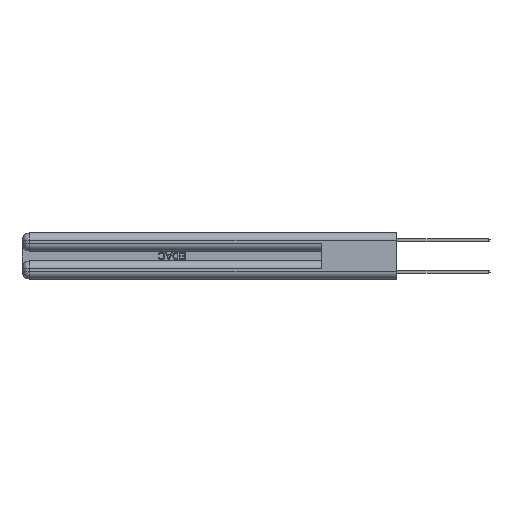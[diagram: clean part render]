
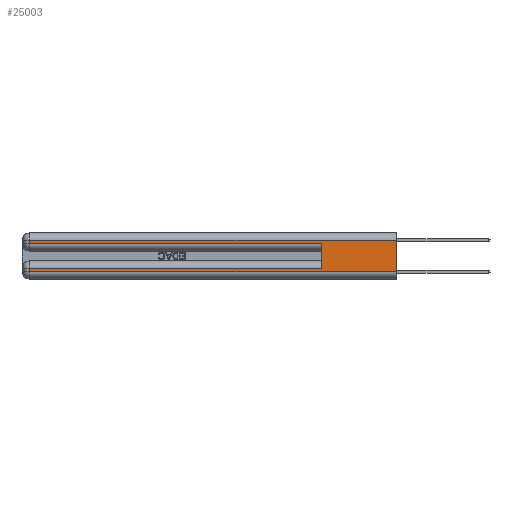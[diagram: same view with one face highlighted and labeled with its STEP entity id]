
A CAD part, left-side view. The second image highlights one B-rep face of the part: STEP entity #25003.
In plain terms, the highlighted planar face has unit normal (-1, 0, 0).
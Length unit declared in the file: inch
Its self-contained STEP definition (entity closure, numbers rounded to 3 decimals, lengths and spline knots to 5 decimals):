
#69 = EDGE_CURVE ( 'NONE', #13166, #26207, #18039, .T. ) ;
#196 = LINE ( 'NONE', #12963, #21649 ) ;
#398 = ORIENTED_EDGE ( 'NONE', *, *, #14017, .T. ) ;
#1386 = VECTOR ( 'NONE', #12212, 39.37008 ) ;
#2842 = EDGE_CURVE ( 'NONE', #34688, #3847, #20074, .T. ) ;
#3004 = CARTESIAN_POINT ( 'NONE',  ( 0., 0., 0.37 ) ) ;
#3355 = VERTEX_POINT ( 'NONE', #21609 ) ;
#3847 = VERTEX_POINT ( 'NONE', #7056 ) ;
#3893 = LINE ( 'NONE', #34822, #27966 ) ;
#4343 = CARTESIAN_POINT ( 'NONE',  ( 0., 2.94, 0.37 ) ) ;
#4474 = VECTOR ( 'NONE', #12182, 39.37008 ) ;
#4668 = ORIENTED_EDGE ( 'NONE', *, *, #28857, .T. ) ;
#5489 = ORIENTED_EDGE ( 'NONE', *, *, #69, .T. ) ;
#5507 = ORIENTED_EDGE ( 'NONE', *, *, #9092, .F. ) ;
#7005 = LINE ( 'NONE', #7199, #21904 ) ;
#7056 = CARTESIAN_POINT ( 'NONE',  ( 0., 0.6, 0.285 ) ) ;
#7199 = CARTESIAN_POINT ( 'NONE',  ( 0., 2.94, 0.37 ) ) ;
#7301 = CARTESIAN_POINT ( 'NONE',  ( 0., 2.94, 0.31 ) ) ;
#7605 = ORIENTED_EDGE ( 'NONE', *, *, #8322, .T. ) ;
#8322 = EDGE_CURVE ( 'NONE', #13550, #3847, #3893, .T. ) ;
#9092 = EDGE_CURVE ( 'NONE', #3355, #11213, #24401, .T. ) ;
#9249 = ORIENTED_EDGE ( 'NONE', *, *, #18118, .T. ) ;
#9753 = FACE_OUTER_BOUND ( 'NONE', #30734, .T. ) ;
#9813 = DIRECTION ( 'NONE',  ( 0., 0., -1. ) ) ;
#11213 = VERTEX_POINT ( 'NONE', #31788 ) ;
#11376 = VECTOR ( 'NONE', #35109, 39.37008 ) ;
#11435 = EDGE_CURVE ( 'NONE', #26207, #11213, #196, .T. ) ;
#11589 = CARTESIAN_POINT ( 'NONE',  ( 0., 0., 0.085 ) ) ;
#12182 = DIRECTION ( 'NONE',  ( 0., 1., 0. ) ) ;
#12212 = DIRECTION ( 'NONE',  ( 0., 0., -1. ) ) ;
#12644 = DIRECTION ( 'NONE',  ( 0., 0., -1. ) ) ;
#12963 = CARTESIAN_POINT ( 'NONE',  ( 0., 0., 0.06 ) ) ;
#13166 = VERTEX_POINT ( 'NONE', #17229 ) ;
#13550 = VERTEX_POINT ( 'NONE', #32478 ) ;
#14017 = EDGE_CURVE ( 'NONE', #27731, #13550, #7005, .T. ) ;
#17229 = CARTESIAN_POINT ( 'NONE',  ( 0., 2.94, 0.085 ) ) ;
#17409 = CARTESIAN_POINT ( 'NONE',  ( 0., 0.6, 0.145 ) ) ;
#18039 = LINE ( 'NONE', #4343, #1386 ) ;
#18118 = EDGE_CURVE ( 'NONE', #3355, #27731, #30698, .T. ) ;
#18136 = CARTESIAN_POINT ( 'NONE',  ( 0., 0., 0.37 ) ) ;
#19317 = CARTESIAN_POINT ( 'NONE',  ( 0., 0., 0.31 ) ) ;
#20074 = LINE ( 'NONE', #17409, #11376 ) ;
#20888 = VECTOR ( 'NONE', #9813, 39.37008 ) ;
#21069 = DIRECTION ( 'NONE',  ( 1., 0., 0. ) ) ;
#21478 = DIRECTION ( 'NONE',  ( 0., -1., 0. ) ) ;
#21609 = CARTESIAN_POINT ( 'NONE',  ( 0., 0., 0.31 ) ) ;
#21649 = VECTOR ( 'NONE', #21478, 39.37008 ) ;
#21904 = VECTOR ( 'NONE', #12644, 39.37008 ) ;
#21994 = LINE ( 'NONE', #11589, #4474 ) ;
#22251 = DIRECTION ( 'NONE',  ( 0., 1., 0. ) ) ;
#22323 = AXIS2_PLACEMENT_3D ( 'NONE', #3004, #21069, #29507 ) ;
#24401 = LINE ( 'NONE', #18136, #20888 ) ;
#25003 = ADVANCED_FACE ( 'NONE', ( #9753 ), #30887, .F. ) ;
#25674 = CARTESIAN_POINT ( 'NONE',  ( 0., 2.94, 0.06 ) ) ;
#26207 = VERTEX_POINT ( 'NONE', #25674 ) ;
#27731 = VERTEX_POINT ( 'NONE', #7301 ) ;
#27966 = VECTOR ( 'NONE', #29054, 39.37008 ) ;
#28857 = EDGE_CURVE ( 'NONE', #34688, #13166, #21994, .T. ) ;
#28983 = ORIENTED_EDGE ( 'NONE', *, *, #2842, .F. ) ;
#29054 = DIRECTION ( 'NONE',  ( 0., -1., 0. ) ) ;
#29507 = DIRECTION ( 'NONE',  ( 0., 0., -1. ) ) ;
#29814 = VECTOR ( 'NONE', #22251, 39.37008 ) ;
#30698 = LINE ( 'NONE', #19317, #29814 ) ;
#30734 = EDGE_LOOP ( 'NONE', ( #5507, #9249, #398, #7605, #28983, #4668, #5489, #33679 ) ) ;
#30887 = PLANE ( 'NONE',  #22323 ) ;
#31788 = CARTESIAN_POINT ( 'NONE',  ( 0., 0., 0.06 ) ) ;
#32478 = CARTESIAN_POINT ( 'NONE',  ( 0., 2.94, 0.285 ) ) ;
#33679 = ORIENTED_EDGE ( 'NONE', *, *, #11435, .T. ) ;
#34688 = VERTEX_POINT ( 'NONE', #35673 ) ;
#34822 = CARTESIAN_POINT ( 'NONE',  ( 0., 0., 0.285 ) ) ;
#35109 = DIRECTION ( 'NONE',  ( 0., 0., 1. ) ) ;
#35673 = CARTESIAN_POINT ( 'NONE',  ( 0., 0.6, 0.085 ) ) ;
